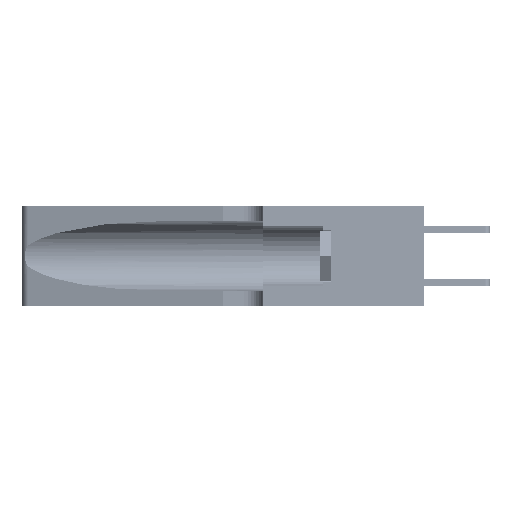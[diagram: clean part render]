
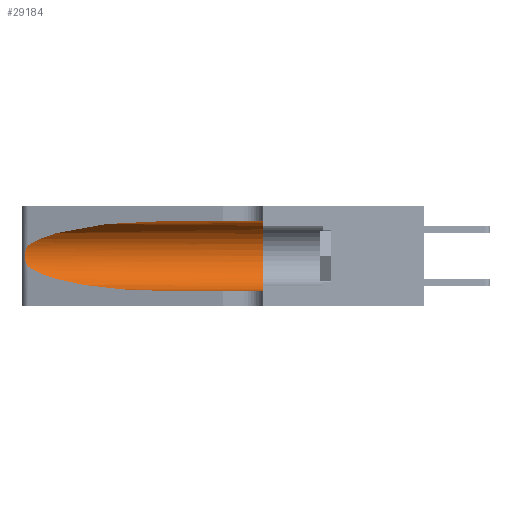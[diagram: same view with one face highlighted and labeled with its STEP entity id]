
A CAD part, left-side view. The second image highlights one B-rep face of the part: STEP entity #29184.
In plain terms, the highlighted cylindrical face has radius 3.308 mm (diameter 6.617 mm), a partial arc.
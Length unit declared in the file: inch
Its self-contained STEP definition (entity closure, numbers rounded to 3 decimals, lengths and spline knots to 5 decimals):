
#1498 =( BOUNDED_CURVE ( )  B_SPLINE_CURVE ( 3, ( #13743, #3396, #34683, #38146 ),
 .UNSPECIFIED., .F., .T. ) 
 B_SPLINE_CURVE_WITH_KNOTS ( ( 4, 4 ),
 ( 1.5708, 2.84003 ),
 .UNSPECIFIED. ) 
 CURVE ( )  GEOMETRIC_REPRESENTATION_ITEM ( )  RATIONAL_B_SPLINE_CURVE ( ( 1., 0.87, 0.87, 1. ) ) 
 REPRESENTATION_ITEM ( '' )  );
#1934 = VERTEX_POINT ( 'NONE', #30486 ) ;
#2349 = LINE ( 'NONE', #29934, #42359 ) ;
#2514 = DIRECTION ( 'NONE',  ( 0., -1., 0. ) ) ;
#2626 = CARTESIAN_POINT ( 'NONE',  ( 0.25487, 1.22718, 0.22369 ) ) ;
#2809 = CARTESIAN_POINT ( 'NONE',  ( 0.25787, 1.23484, 0.2124 ) ) ;
#3396 = CARTESIAN_POINT ( 'NONE',  ( 0.18966, 0.96281, 0.31525 ) ) ;
#3491 = CARTESIAN_POINT ( 'NONE',  ( 0.1305, 0.35, 0.05475 ) ) ;
#4205 = CARTESIAN_POINT ( 'NONE',  ( 0.25555, 1.22993, 0.14849 ) ) ;
#6321 = B_SPLINE_CURVE_WITH_KNOTS ( 'NONE', 3,
 ( #40147, #36964, #13602, #2809, #44396, #27478, #13148, #9946, #42430, #10900, #18158, #41831, #4205, #21338 ),
 .UNSPECIFIED., .F., .F.,
 ( 4, 2, 2, 2, 2, 2, 4 ),
 ( 0., 0.00027, 0.00053, 0.00107, 0.0016, 0.00187, 0.00214 ),
 .UNSPECIFIED. ) ;
#6768 = EDGE_LOOP ( 'NONE', ( #28338, #40871, #22693, #38020, #29724, #35919 ) ) ;
#9043 = CARTESIAN_POINT ( 'NONE',  ( 0.25487, 1.22718, 0.14631 ) ) ;
#9618 = VERTEX_POINT ( 'NONE', #33911 ) ;
#9629 = LINE ( 'NONE', #31569, #36592 ) ;
#9946 = CARTESIAN_POINT ( 'NONE',  ( 0.26075, 1.23896, 0.178 ) ) ;
#10794 = DIRECTION ( 'NONE',  ( 0., -1., 0. ) ) ;
#10900 = CARTESIAN_POINT ( 'NONE',  ( 0.25856, 1.23593, 0.16098 ) ) ;
#12193 = CIRCLE ( 'NONE', #41483, 0.13025 ) ;
#12329 = EDGE_CURVE ( 'NONE', #1934, #15254, #9629, .T. ) ;
#12514 = CARTESIAN_POINT ( 'NONE',  ( 0.1305, 1.61858, 0.185 ) ) ;
#13148 = CARTESIAN_POINT ( 'NONE',  ( 0.26075, 1.23896, 0.19203 ) ) ;
#13267 = CARTESIAN_POINT ( 'NONE',  ( 0.1305, 0.35, 0.185 ) ) ;
#13602 = CARTESIAN_POINT ( 'NONE',  ( 0.25639, 1.23184, 0.21858 ) ) ;
#13743 = CARTESIAN_POINT ( 'NONE',  ( 0.1305, 0.72297, 0.31525 ) ) ;
#15254 = VERTEX_POINT ( 'NONE', #3491 ) ;
#16024 = CARTESIAN_POINT ( 'NONE',  ( 0.2373, 1.15595, 0.08982 ) ) ;
#16170 = CARTESIAN_POINT ( 'NONE',  ( 0.18966, 0.96281, 0.05475 ) ) ;
#18158 = CARTESIAN_POINT ( 'NONE',  ( 0.25789, 1.23486, 0.15765 ) ) ;
#19101 =( BOUNDED_CURVE ( )  B_SPLINE_CURVE ( 3, ( #9043, #16024, #16170, #30040 ),
 .UNSPECIFIED., .F., .T. ) 
 B_SPLINE_CURVE_WITH_KNOTS ( ( 4, 4 ),
 ( 3.44316, 4.71239 ),
 .UNSPECIFIED. ) 
 CURVE ( )  GEOMETRIC_REPRESENTATION_ITEM ( )  RATIONAL_B_SPLINE_CURVE ( ( 1., 0.87, 0.87, 1. ) ) 
 REPRESENTATION_ITEM ( '' )  );
#20067 = DIRECTION ( 'NONE',  ( 0., 1., 0. ) ) ;
#21338 = CARTESIAN_POINT ( 'NONE',  ( 0.25487, 1.22718, 0.14631 ) ) ;
#22693 = ORIENTED_EDGE ( 'NONE', *, *, #35023, .T. ) ;
#24212 = EDGE_CURVE ( 'NONE', #26562, #31820, #1498, .T. ) ;
#25867 = DIRECTION ( 'NONE',  ( 0., -1., 0. ) ) ;
#26461 = EDGE_CURVE ( 'NONE', #31820, #9618, #6321, .T. ) ;
#26562 = VERTEX_POINT ( 'NONE', #31945 ) ;
#27478 = CARTESIAN_POINT ( 'NONE',  ( 0.26018, 1.23835, 0.19895 ) ) ;
#28338 = ORIENTED_EDGE ( 'NONE', *, *, #24212, .T. ) ;
#29184 = ADVANCED_FACE ( 'NONE', ( #35791 ), #32001, .F. ) ;
#29724 = ORIENTED_EDGE ( 'NONE', *, *, #43671, .F. ) ;
#29934 = CARTESIAN_POINT ( 'NONE',  ( 0.1305, 1.61858, 0.31525 ) ) ;
#30040 = CARTESIAN_POINT ( 'NONE',  ( 0.1305, 0.72297, 0.05475 ) ) ;
#30486 = CARTESIAN_POINT ( 'NONE',  ( 0.1305, 0.72297, 0.05475 ) ) ;
#31569 = CARTESIAN_POINT ( 'NONE',  ( 0.1305, 1.61858, 0.05475 ) ) ;
#31820 = VERTEX_POINT ( 'NONE', #2626 ) ;
#31945 = CARTESIAN_POINT ( 'NONE',  ( 0.1305, 0.72297, 0.31525 ) ) ;
#32001 = CYLINDRICAL_SURFACE ( 'NONE', #44086, 0.13025 ) ;
#33911 = CARTESIAN_POINT ( 'NONE',  ( 0.25487, 1.22718, 0.14631 ) ) ;
#34374 = VERTEX_POINT ( 'NONE', #38926 ) ;
#34394 = EDGE_CURVE ( 'NONE', #26562, #34374, #2349, .T. ) ;
#34683 = CARTESIAN_POINT ( 'NONE',  ( 0.2373, 1.15595, 0.28018 ) ) ;
#35023 = EDGE_CURVE ( 'NONE', #9618, #1934, #19101, .T. ) ;
#35791 = FACE_OUTER_BOUND ( 'NONE', #6768, .T. ) ;
#35919 = ORIENTED_EDGE ( 'NONE', *, *, #34394, .F. ) ;
#36592 = VECTOR ( 'NONE', #25867, 39.37008 ) ;
#36903 = DIRECTION ( 'NONE',  ( 0., 0., -1. ) ) ;
#36964 = CARTESIAN_POINT ( 'NONE',  ( 0.25555, 1.22994, 0.2215 ) ) ;
#38020 = ORIENTED_EDGE ( 'NONE', *, *, #12329, .T. ) ;
#38146 = CARTESIAN_POINT ( 'NONE',  ( 0.25487, 1.22718, 0.22369 ) ) ;
#38926 = CARTESIAN_POINT ( 'NONE',  ( 0.1305, 0.35, 0.31525 ) ) ;
#40147 = CARTESIAN_POINT ( 'NONE',  ( 0.25487, 1.22718, 0.22369 ) ) ;
#40871 = ORIENTED_EDGE ( 'NONE', *, *, #26461, .T. ) ;
#41483 = AXIS2_PLACEMENT_3D ( 'NONE', #13267, #20067, #43899 ) ;
#41831 = CARTESIAN_POINT ( 'NONE',  ( 0.25639, 1.23186, 0.15144 ) ) ;
#42359 = VECTOR ( 'NONE', #2514, 39.37008 ) ;
#42430 = CARTESIAN_POINT ( 'NONE',  ( 0.26017, 1.23833, 0.17102 ) ) ;
#43671 = EDGE_CURVE ( 'NONE', #34374, #15254, #12193, .T. ) ;
#43899 = DIRECTION ( 'NONE',  ( 0., 0., 1. ) ) ;
#44086 = AXIS2_PLACEMENT_3D ( 'NONE', #12514, #10794, #36903 ) ;
#44396 = CARTESIAN_POINT ( 'NONE',  ( 0.25854, 1.2359, 0.20912 ) ) ;
